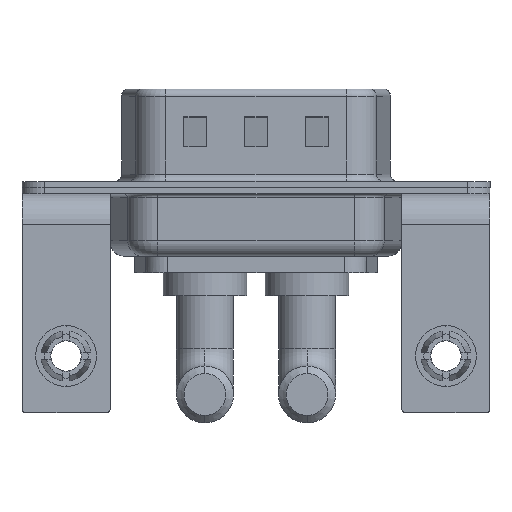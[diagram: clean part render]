
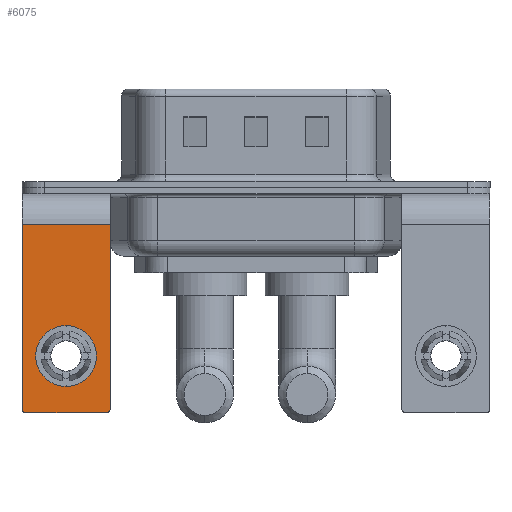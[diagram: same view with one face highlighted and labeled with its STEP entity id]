
A CAD part, front view. The second image highlights one B-rep face of the part: STEP entity #6075.
In plain terms, the highlighted planar face has unit normal (0, -1, 0).
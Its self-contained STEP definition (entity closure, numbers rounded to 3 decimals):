
#159 = CARTESIAN_POINT ( 'NONE',  ( 2.9, -6.25, -14.55 ) ) ;
#270 = ORIENTED_EDGE ( 'NONE', *, *, #8435, .T. ) ;
#490 = CARTESIAN_POINT ( 'NONE',  ( 0., -6.25, -11.07 ) ) ;
#562 = EDGE_CURVE ( 'NONE', #13128, #832, #1063, .T. ) ;
#832 = VERTEX_POINT ( 'NONE', #2984 ) ;
#1061 = CARTESIAN_POINT ( 'NONE',  ( -2.9, -6.25, -2.4 ) ) ;
#1063 = CIRCLE ( 'NONE', #3225, 0.25 ) ;
#1523 = DIRECTION ( 'NONE',  ( 0., 0., 1. ) ) ;
#1575 = DIRECTION ( 'NONE',  ( 0., 1., 0. ) ) ;
#2033 = CARTESIAN_POINT ( 'NONE',  ( 2.9, -6.25, -2.4 ) ) ;
#2188 = VERTEX_POINT ( 'NONE', #2379 ) ;
#2371 = ORIENTED_EDGE ( 'NONE', *, *, #4840, .T. ) ;
#2379 = CARTESIAN_POINT ( 'NONE',  ( 0., -6.25, -13.07 ) ) ;
#2427 = CARTESIAN_POINT ( 'NONE',  ( 2.9, -6.25, -2.4 ) ) ;
#2675 = CARTESIAN_POINT ( 'NONE',  ( 2.65, -6.25, -14.55 ) ) ;
#2799 = CIRCLE ( 'NONE', #13335, 0.25 ) ;
#2984 = CARTESIAN_POINT ( 'NONE',  ( -2.65, -6.25, -14.8 ) ) ;
#3072 = EDGE_LOOP ( 'NONE', ( #270, #10842, #13340, #8919, #13812, #15936 ) ) ;
#3215 = AXIS2_PLACEMENT_3D ( 'NONE', #2427, #1575, #15982 ) ;
#3225 = AXIS2_PLACEMENT_3D ( 'NONE', #14846, #9485, #5783 ) ;
#3231 = VERTEX_POINT ( 'NONE', #15367 ) ;
#3819 = CARTESIAN_POINT ( 'NONE',  ( -2.9, -6.25, -2.4 ) ) ;
#4682 = EDGE_CURVE ( 'NONE', #9753, #7435, #2799, .T. ) ;
#4840 = EDGE_CURVE ( 'NONE', #2188, #10079, #11792, .T. ) ;
#5003 = EDGE_CURVE ( 'NONE', #9753, #832, #15530, .T. ) ;
#5273 = CARTESIAN_POINT ( 'NONE',  ( 2.9, -6.25, -14.8 ) ) ;
#5582 = CIRCLE ( 'NONE', #14515, 2. ) ;
#5639 = DIRECTION ( 'NONE',  ( 0., 0., 1. ) ) ;
#5783 = DIRECTION ( 'NONE',  ( 0., 0., 1. ) ) ;
#5959 = CARTESIAN_POINT ( 'NONE',  ( -2.9, -6.25, -14.55 ) ) ;
#6075 = ADVANCED_FACE ( 'NONE', ( #10111, #15304 ), #14019, .F. ) ;
#7435 = VERTEX_POINT ( 'NONE', #159 ) ;
#7454 = VECTOR ( 'NONE', #16763, 1000. ) ;
#7678 = DIRECTION ( 'NONE',  ( 0., -1., 0. ) ) ;
#7874 = VERTEX_POINT ( 'NONE', #1061 ) ;
#8435 = EDGE_CURVE ( 'NONE', #7874, #13128, #15434, .T. ) ;
#8539 = DIRECTION ( 'NONE',  ( -1., 0., 0. ) ) ;
#8642 = CARTESIAN_POINT ( 'NONE',  ( 2.65, -6.25, -14.8 ) ) ;
#8919 = ORIENTED_EDGE ( 'NONE', *, *, #4682, .T. ) ;
#8941 = DIRECTION ( 'NONE',  ( 0., 0., 1. ) ) ;
#8985 = DIRECTION ( 'NONE',  ( 0., 0., -1. ) ) ;
#9082 = DIRECTION ( 'NONE',  ( -1., 0., 0. ) ) ;
#9298 = EDGE_LOOP ( 'NONE', ( #2371, #11060 ) ) ;
#9485 = DIRECTION ( 'NONE',  ( 0., -1., 0. ) ) ;
#9549 = DIRECTION ( 'NONE',  ( 0., 1., 0. ) ) ;
#9753 = VERTEX_POINT ( 'NONE', #8642 ) ;
#10079 = VERTEX_POINT ( 'NONE', #15745 ) ;
#10111 = FACE_BOUND ( 'NONE', #9298, .T. ) ;
#10198 = LINE ( 'NONE', #11377, #7454 ) ;
#10842 = ORIENTED_EDGE ( 'NONE', *, *, #562, .T. ) ;
#11060 = ORIENTED_EDGE ( 'NONE', *, *, #15749, .T. ) ;
#11350 = VECTOR ( 'NONE', #8985, 1000. ) ;
#11377 = CARTESIAN_POINT ( 'NONE',  ( 2.9, -6.25, -2.4 ) ) ;
#11754 = CARTESIAN_POINT ( 'NONE',  ( 0., -6.25, -11.07 ) ) ;
#11792 = CIRCLE ( 'NONE', #15319, 2. ) ;
#12094 = LINE ( 'NONE', #2033, #14806 ) ;
#13128 = VERTEX_POINT ( 'NONE', #5959 ) ;
#13335 = AXIS2_PLACEMENT_3D ( 'NONE', #2675, #7678, #8941 ) ;
#13340 = ORIENTED_EDGE ( 'NONE', *, *, #5003, .F. ) ;
#13368 = VECTOR ( 'NONE', #9082, 1000. ) ;
#13812 = ORIENTED_EDGE ( 'NONE', *, *, #14617, .F. ) ;
#14019 = PLANE ( 'NONE',  #3215 ) ;
#14515 = AXIS2_PLACEMENT_3D ( 'NONE', #11754, #9549, #1523 ) ;
#14617 = EDGE_CURVE ( 'NONE', #3231, #7435, #10198, .T. ) ;
#14806 = VECTOR ( 'NONE', #8539, 1000. ) ;
#14846 = CARTESIAN_POINT ( 'NONE',  ( -2.65, -6.25, -14.55 ) ) ;
#15304 = FACE_OUTER_BOUND ( 'NONE', #3072, .T. ) ;
#15319 = AXIS2_PLACEMENT_3D ( 'NONE', #490, #15896, #5639 ) ;
#15367 = CARTESIAN_POINT ( 'NONE',  ( 2.9, -6.25, -2.4 ) ) ;
#15434 = LINE ( 'NONE', #3819, #11350 ) ;
#15530 = LINE ( 'NONE', #5273, #13368 ) ;
#15745 = CARTESIAN_POINT ( 'NONE',  ( 0., -6.25, -9.07 ) ) ;
#15749 = EDGE_CURVE ( 'NONE', #10079, #2188, #5582, .T. ) ;
#15858 = EDGE_CURVE ( 'NONE', #3231, #7874, #12094, .T. ) ;
#15896 = DIRECTION ( 'NONE',  ( 0., 1., 0. ) ) ;
#15936 = ORIENTED_EDGE ( 'NONE', *, *, #15858, .T. ) ;
#15982 = DIRECTION ( 'NONE',  ( 0., 0., 1. ) ) ;
#16763 = DIRECTION ( 'NONE',  ( 0., 0., -1. ) ) ;
